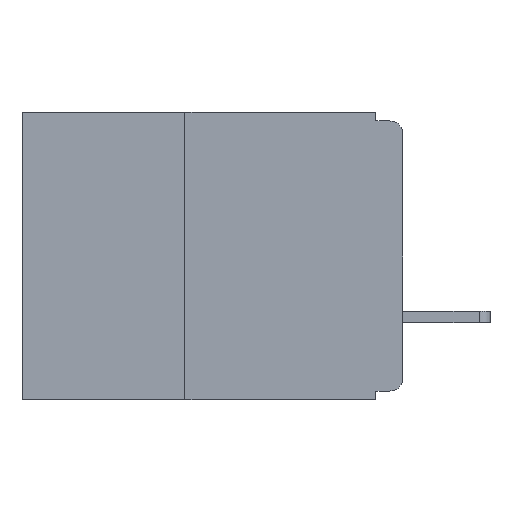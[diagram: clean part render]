
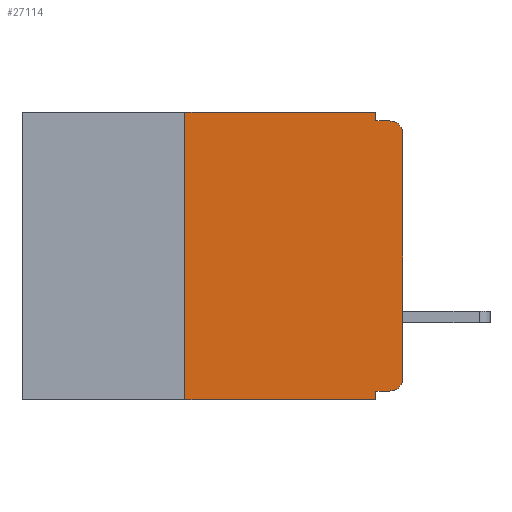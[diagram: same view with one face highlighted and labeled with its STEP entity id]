
A CAD part, left-side view. The second image highlights one B-rep face of the part: STEP entity #27114.
In plain terms, the highlighted planar face has unit normal (-1, 0, 0).
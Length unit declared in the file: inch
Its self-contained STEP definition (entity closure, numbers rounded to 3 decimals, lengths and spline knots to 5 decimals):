
#322 = VECTOR ( 'NONE', #18069, 39.37008 ) ;
#532 = FACE_OUTER_BOUND ( 'NONE', #27088, .T. ) ;
#715 = CARTESIAN_POINT ( 'NONE',  ( 0., 0.031, -0.01 ) ) ;
#788 = CARTESIAN_POINT ( 'NONE',  ( 0., 0.437, 0. ) ) ;
#1967 = DIRECTION ( 'NONE',  ( -1., 0., 0. ) ) ;
#2255 = VERTEX_POINT ( 'NONE', #18042 ) ;
#2325 = VECTOR ( 'NONE', #27156, 39.37008 ) ;
#2573 = CARTESIAN_POINT ( 'NONE',  ( 0., 0.437, 0. ) ) ;
#3382 = EDGE_CURVE ( 'NONE', #10084, #24869, #15809, .T. ) ;
#4234 = EDGE_CURVE ( 'NONE', #15738, #10084, #24290, .T. ) ;
#4302 = LINE ( 'NONE', #15479, #23599 ) ;
#4365 = CARTESIAN_POINT ( 'NONE',  ( 0., 0.015, -0.025 ) ) ;
#4368 = CIRCLE ( 'NONE', #33257, 0.015 ) ;
#4417 = CARTESIAN_POINT ( 'NONE',  ( 0., 0.031, -0.33 ) ) ;
#5337 = DIRECTION ( 'NONE',  ( 0., 0., -1. ) ) ;
#7025 = DIRECTION ( 'NONE',  ( 0., 0., -1. ) ) ;
#7420 = CARTESIAN_POINT ( 'NONE',  ( 0., 0.015, -0.32 ) ) ;
#7685 = AXIS2_PLACEMENT_3D ( 'NONE', #2573, #21044, #5337 ) ;
#9069 = CIRCLE ( 'NONE', #19357, 0.015 ) ;
#9163 = DIRECTION ( 'NONE',  ( 0., -1., 0. ) ) ;
#9507 = LINE ( 'NONE', #16769, #2325 ) ;
#9673 = VECTOR ( 'NONE', #32604, 39.37008 ) ;
#10084 = VERTEX_POINT ( 'NONE', #23709 ) ;
#10741 = ORIENTED_EDGE ( 'NONE', *, *, #15584, .T. ) ;
#11945 = EDGE_CURVE ( 'NONE', #23918, #24774, #18886, .T. ) ;
#12605 = VERTEX_POINT ( 'NONE', #715 ) ;
#12953 = CARTESIAN_POINT ( 'NONE',  ( 0., 0., -0.32 ) ) ;
#14049 = DIRECTION ( 'NONE',  ( 0., 0., 1. ) ) ;
#14075 = DIRECTION ( 'NONE',  ( 0., 0., 1. ) ) ;
#14615 = ORIENTED_EDGE ( 'NONE', *, *, #11945, .T. ) ;
#14639 = EDGE_CURVE ( 'NONE', #26176, #2255, #20584, .T. ) ;
#15047 = CARTESIAN_POINT ( 'NONE',  ( 0., 0.031, 0. ) ) ;
#15313 = CARTESIAN_POINT ( 'NONE',  ( 0., 0.25, -0.33 ) ) ;
#15479 = CARTESIAN_POINT ( 'NONE',  ( 0., 0.031, 0. ) ) ;
#15584 = EDGE_CURVE ( 'NONE', #15738, #24356, #9507, .T. ) ;
#15630 = EDGE_CURVE ( 'NONE', #2255, #24356, #30159, .T. ) ;
#15738 = VERTEX_POINT ( 'NONE', #30366 ) ;
#15809 = LINE ( 'NONE', #788, #9673 ) ;
#15813 = EDGE_CURVE ( 'NONE', #24774, #22238, #9069, .T. ) ;
#16363 = ORIENTED_EDGE ( 'NONE', *, *, #15813, .T. ) ;
#16769 = CARTESIAN_POINT ( 'NONE',  ( 0., 0.437, -0.33 ) ) ;
#17379 = VECTOR ( 'NONE', #14049, 39.37008 ) ;
#17858 = CARTESIAN_POINT ( 'NONE',  ( 0., 0.015, -0.305 ) ) ;
#18042 = CARTESIAN_POINT ( 'NONE',  ( 0., 0.031, -0.32 ) ) ;
#18069 = DIRECTION ( 'NONE',  ( 0., 1., 0. ) ) ;
#18074 = DIRECTION ( 'NONE',  ( 0., 0., -1. ) ) ;
#18439 = PLANE ( 'NONE',  #7685 ) ;
#18721 = ORIENTED_EDGE ( 'NONE', *, *, #3382, .F. ) ;
#18886 = LINE ( 'NONE', #21895, #25745 ) ;
#19357 = AXIS2_PLACEMENT_3D ( 'NONE', #4365, #22727, #7025 ) ;
#19600 = CARTESIAN_POINT ( 'NONE',  ( 0., 0.031, -0.33 ) ) ;
#19969 = ORIENTED_EDGE ( 'NONE', *, *, #14639, .F. ) ;
#20455 = DIRECTION ( 'NONE',  ( 0., 0., -1. ) ) ;
#20584 = LINE ( 'NONE', #12953, #322 ) ;
#21044 = DIRECTION ( 'NONE',  ( 1., 0., 0. ) ) ;
#21739 = VECTOR ( 'NONE', #22090, 39.37008 ) ;
#21895 = CARTESIAN_POINT ( 'NONE',  ( 0., 0., 0. ) ) ;
#22077 = ORIENTED_EDGE ( 'NONE', *, *, #33688, .F. ) ;
#22090 = DIRECTION ( 'NONE',  ( 0., 0., -1. ) ) ;
#22158 = CARTESIAN_POINT ( 'NONE',  ( 0., 0., -0.01 ) ) ;
#22238 = VERTEX_POINT ( 'NONE', #25971 ) ;
#22498 = CARTESIAN_POINT ( 'NONE',  ( 0., 0., -0.305 ) ) ;
#22727 = DIRECTION ( 'NONE',  ( -1., 0., 0. ) ) ;
#23599 = VECTOR ( 'NONE', #18074, 39.37008 ) ;
#23709 = CARTESIAN_POINT ( 'NONE',  ( 0., 0.25, 0. ) ) ;
#23918 = VERTEX_POINT ( 'NONE', #22498 ) ;
#24290 = LINE ( 'NONE', #15313, #17379 ) ;
#24356 = VERTEX_POINT ( 'NONE', #4417 ) ;
#24711 = ORIENTED_EDGE ( 'NONE', *, *, #15630, .F. ) ;
#24774 = VERTEX_POINT ( 'NONE', #29688 ) ;
#24869 = VERTEX_POINT ( 'NONE', #15047 ) ;
#25606 = VECTOR ( 'NONE', #9163, 39.37008 ) ;
#25745 = VECTOR ( 'NONE', #14075, 39.37008 ) ;
#25971 = CARTESIAN_POINT ( 'NONE',  ( 0., 0.015, -0.01 ) ) ;
#26176 = VERTEX_POINT ( 'NONE', #7420 ) ;
#26790 = EDGE_CURVE ( 'NONE', #26176, #23918, #4368, .T. ) ;
#26796 = ORIENTED_EDGE ( 'NONE', *, *, #26790, .T. ) ;
#27088 = EDGE_LOOP ( 'NONE', ( #14615, #16363, #22077, #32752, #18721, #30580, #10741, #24711, #19969, #26796 ) ) ;
#27114 = ADVANCED_FACE ( 'NONE', ( #532 ), #18439, .F. ) ;
#27156 = DIRECTION ( 'NONE',  ( 0., -1., 0. ) ) ;
#27609 = EDGE_CURVE ( 'NONE', #24869, #12605, #4302, .T. ) ;
#29688 = CARTESIAN_POINT ( 'NONE',  ( 0., 0., -0.025 ) ) ;
#30159 = LINE ( 'NONE', #19600, #21739 ) ;
#30366 = CARTESIAN_POINT ( 'NONE',  ( 0., 0.25, -0.33 ) ) ;
#30580 = ORIENTED_EDGE ( 'NONE', *, *, #4234, .F. ) ;
#32373 = LINE ( 'NONE', #22158, #25606 ) ;
#32604 = DIRECTION ( 'NONE',  ( 0., -1., 0. ) ) ;
#32752 = ORIENTED_EDGE ( 'NONE', *, *, #27609, .F. ) ;
#33257 = AXIS2_PLACEMENT_3D ( 'NONE', #17858, #1967, #20455 ) ;
#33688 = EDGE_CURVE ( 'NONE', #12605, #22238, #32373, .T. ) ;
